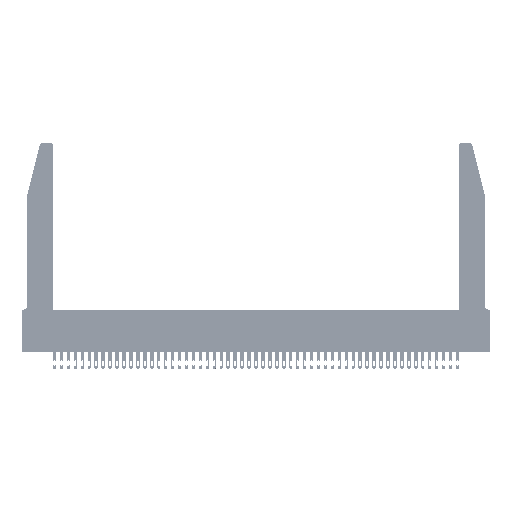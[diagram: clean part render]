
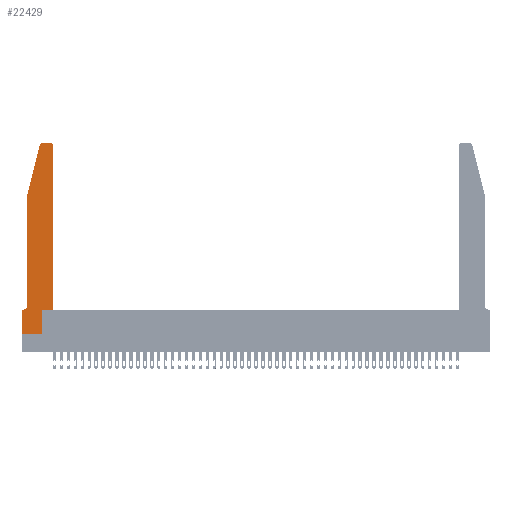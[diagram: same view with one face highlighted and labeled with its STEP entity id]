
A CAD part, top view. The second image highlights one B-rep face of the part: STEP entity #22429.
In plain terms, the highlighted planar face has unit normal (0, 0, 1).
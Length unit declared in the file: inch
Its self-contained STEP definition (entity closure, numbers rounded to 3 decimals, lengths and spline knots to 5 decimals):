
#974 = LINE ( 'NONE', #14465, #5717 ) ;
#1148 = EDGE_CURVE ( 'NONE', #4275, #18563, #11451, .T. ) ;
#1582 = VERTEX_POINT ( 'NONE', #29131 ) ;
#2688 = EDGE_CURVE ( 'NONE', #1582, #16519, #33029, .T. ) ;
#2808 = DIRECTION ( 'NONE',  ( 0., 0., 1. ) ) ;
#3454 = CARTESIAN_POINT ( 'NONE',  ( 0.25487, 2.72718, 0.37 ) ) ;
#3701 = ORIENTED_EDGE ( 'NONE', *, *, #17720, .T. ) ;
#3999 = VERTEX_POINT ( 'NONE', #3454 ) ;
#4275 = VERTEX_POINT ( 'NONE', #25183 ) ;
#5202 = AXIS2_PLACEMENT_3D ( 'NONE', #6592, #40759, #48307 ) ;
#5697 = EDGE_CURVE ( 'NONE', #10413, #38580, #974, .T. ) ;
#5717 = VECTOR ( 'NONE', #14803, 39.37008 ) ;
#6514 = CARTESIAN_POINT ( 'NONE',  ( 0., 0., 0.37 ) ) ;
#6592 = CARTESIAN_POINT ( 'NONE',  ( 0.0055, 0.42, 0.37 ) ) ;
#6845 = DIRECTION ( 'NONE',  ( -0.239, -0.971, 0. ) ) ;
#7261 = ORIENTED_EDGE ( 'NONE', *, *, #48151, .T. ) ;
#7320 = CARTESIAN_POINT ( 'NONE',  ( 0.2865, 0.35, 0.37 ) ) ;
#7321 = ORIENTED_EDGE ( 'NONE', *, *, #44157, .T. ) ;
#7394 = VECTOR ( 'NONE', #10785, 39.37008 ) ;
#7941 = PLANE ( 'NONE',  #35559 ) ;
#7947 = LINE ( 'NONE', #7320, #7394 ) ;
#8229 = EDGE_CURVE ( 'NONE', #31064, #19152, #35942, .T. ) ;
#8467 = CARTESIAN_POINT ( 'NONE',  ( 0.0755, 0.35, 0.37 ) ) ;
#9562 = CARTESIAN_POINT ( 'NONE',  ( 0., 0., 0.37 ) ) ;
#10065 = VECTOR ( 'NONE', #32780, 39.37008 ) ;
#10413 = VERTEX_POINT ( 'NONE', #45693 ) ;
#10737 = CARTESIAN_POINT ( 'NONE',  ( 0.0755, 0.42, 0.37 ) ) ;
#10781 = ORIENTED_EDGE ( 'NONE', *, *, #40978, .T. ) ;
#10785 = DIRECTION ( 'NONE',  ( 0., 1., 0. ) ) ;
#11451 = CIRCLE ( 'NONE', #15899, 0.03 ) ;
#11577 = ORIENTED_EDGE ( 'NONE', *, *, #31099, .T. ) ;
#12595 = DIRECTION ( 'NONE',  ( 1., 0., 0. ) ) ;
#12767 = CARTESIAN_POINT ( 'NONE',  ( 0.284, 2.75, 0.37 ) ) ;
#13112 = CARTESIAN_POINT ( 'NONE',  ( 0.4505, 0.35, 0.37 ) ) ;
#13444 = VERTEX_POINT ( 'NONE', #26908 ) ;
#14248 = ORIENTED_EDGE ( 'NONE', *, *, #8229, .T. ) ;
#14465 = CARTESIAN_POINT ( 'NONE',  ( 0.0755, 2., 0.37 ) ) ;
#14803 = DIRECTION ( 'NONE',  ( 0., -1., 0. ) ) ;
#15206 = CARTESIAN_POINT ( 'NONE',  ( 0., 0.35, 0.37 ) ) ;
#15657 = LINE ( 'NONE', #13112, #24490 ) ;
#15725 = CARTESIAN_POINT ( 'NONE',  ( 0.284, 2.72, 0.37 ) ) ;
#15899 = AXIS2_PLACEMENT_3D ( 'NONE', #40273, #2808, #43421 ) ;
#16519 = VERTEX_POINT ( 'NONE', #15206 ) ;
#17196 = DIRECTION ( 'NONE',  ( -1., 0., 0. ) ) ;
#17720 = EDGE_CURVE ( 'NONE', #35572, #3999, #32673, .T. ) ;
#17772 = VERTEX_POINT ( 'NONE', #34644 ) ;
#18563 = VERTEX_POINT ( 'NONE', #19913 ) ;
#19137 = AXIS2_PLACEMENT_3D ( 'NONE', #15725, #39039, #42493 ) ;
#19152 = VERTEX_POINT ( 'NONE', #42724 ) ;
#19369 = ORIENTED_EDGE ( 'NONE', *, *, #5697, .T. ) ;
#19591 = CARTESIAN_POINT ( 'NONE',  ( 0.4505, 0.35, 0.37 ) ) ;
#19835 = DIRECTION ( 'NONE',  ( 0., 0., 1. ) ) ;
#19913 = CARTESIAN_POINT ( 'NONE',  ( 0.4205, 2.75, 0.37 ) ) ;
#20314 = VECTOR ( 'NONE', #38055, 39.37008 ) ;
#20634 = CARTESIAN_POINT ( 'NONE',  ( 0.0755, 2., 0.37 ) ) ;
#22058 = ORIENTED_EDGE ( 'NONE', *, *, #2688, .T. ) ;
#22429 = ADVANCED_FACE ( 'NONE', ( #36373 ), #7941, .T. ) ;
#22740 = EDGE_CURVE ( 'NONE', #17772, #4275, #36990, .T. ) ;
#24191 = VECTOR ( 'NONE', #17196, 39.37008 ) ;
#24490 = VECTOR ( 'NONE', #12595, 39.37008 ) ;
#25183 = CARTESIAN_POINT ( 'NONE',  ( 0.4505, 2.72, 0.37 ) ) ;
#26908 = CARTESIAN_POINT ( 'NONE',  ( 0.2865, 0.35, 0.37 ) ) ;
#27757 = LINE ( 'NONE', #32260, #24191 ) ;
#28388 = ORIENTED_EDGE ( 'NONE', *, *, #1148, .T. ) ;
#29131 = CARTESIAN_POINT ( 'NONE',  ( 0.0055, 0.35, 0.37 ) ) ;
#30826 = EDGE_LOOP ( 'NONE', ( #7261, #3701, #10781, #19369, #11577, #22058, #7321, #14248, #44418, #37286, #46846, #28388 ) ) ;
#31064 = VERTEX_POINT ( 'NONE', #9562 ) ;
#31099 = EDGE_CURVE ( 'NONE', #38580, #1582, #46282, .T. ) ;
#32260 = CARTESIAN_POINT ( 'NONE',  ( 0.2605, 2.75, 0.37 ) ) ;
#32664 = EDGE_CURVE ( 'NONE', #19152, #13444, #7947, .T. ) ;
#32673 = CIRCLE ( 'NONE', #19137, 0.03 ) ;
#32780 = DIRECTION ( 'NONE',  ( 1., 0., 0. ) ) ;
#33029 = LINE ( 'NONE', #8467, #37170 ) ;
#34240 = DIRECTION ( 'NONE',  ( 1., 0., 0. ) ) ;
#34472 = DIRECTION ( 'NONE',  ( 0., 1., 0. ) ) ;
#34573 = CARTESIAN_POINT ( 'NONE',  ( 0., 0.35, 0.37 ) ) ;
#34642 = DIRECTION ( 'NONE',  ( -1., 0., 0. ) ) ;
#34644 = CARTESIAN_POINT ( 'NONE',  ( 0.4505, 0.35, 0.37 ) ) ;
#35394 = CARTESIAN_POINT ( 'NONE',  ( 0., 0., 0.37 ) ) ;
#35559 = AXIS2_PLACEMENT_3D ( 'NONE', #34573, #19835, #34240 ) ;
#35568 = EDGE_CURVE ( 'NONE', #13444, #17772, #15657, .T. ) ;
#35572 = VERTEX_POINT ( 'NONE', #12767 ) ;
#35825 = VECTOR ( 'NONE', #34472, 39.37008 ) ;
#35942 = LINE ( 'NONE', #6514, #10065 ) ;
#36373 = FACE_OUTER_BOUND ( 'NONE', #30826, .T. ) ;
#36990 = LINE ( 'NONE', #19591, #35825 ) ;
#37170 = VECTOR ( 'NONE', #34642, 39.37008 ) ;
#37286 = ORIENTED_EDGE ( 'NONE', *, *, #35568, .T. ) ;
#38055 = DIRECTION ( 'NONE',  ( 0., -1., 0. ) ) ;
#38580 = VERTEX_POINT ( 'NONE', #10737 ) ;
#39039 = DIRECTION ( 'NONE',  ( 0., 0., 1. ) ) ;
#40273 = CARTESIAN_POINT ( 'NONE',  ( 0.4205, 2.72, 0.37 ) ) ;
#40759 = DIRECTION ( 'NONE',  ( 0., 0., -1. ) ) ;
#40978 = EDGE_CURVE ( 'NONE', #3999, #10413, #41071, .T. ) ;
#41071 = LINE ( 'NONE', #20634, #48086 ) ;
#42493 = DIRECTION ( 'NONE',  ( 1., 0., 0. ) ) ;
#42724 = CARTESIAN_POINT ( 'NONE',  ( 0.2865, 0., 0.37 ) ) ;
#43421 = DIRECTION ( 'NONE',  ( 1., 0., 0. ) ) ;
#44157 = EDGE_CURVE ( 'NONE', #16519, #31064, #45528, .T. ) ;
#44418 = ORIENTED_EDGE ( 'NONE', *, *, #32664, .T. ) ;
#45528 = LINE ( 'NONE', #35394, #20314 ) ;
#45693 = CARTESIAN_POINT ( 'NONE',  ( 0.0755, 2., 0.37 ) ) ;
#46282 = CIRCLE ( 'NONE', #5202, 0.07 ) ;
#46846 = ORIENTED_EDGE ( 'NONE', *, *, #22740, .T. ) ;
#48086 = VECTOR ( 'NONE', #6845, 39.37008 ) ;
#48151 = EDGE_CURVE ( 'NONE', #18563, #35572, #27757, .T. ) ;
#48307 = DIRECTION ( 'NONE',  ( -1., 0., 0. ) ) ;
